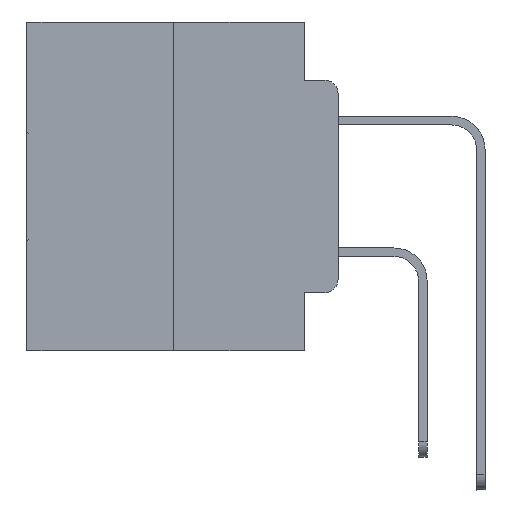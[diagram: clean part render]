
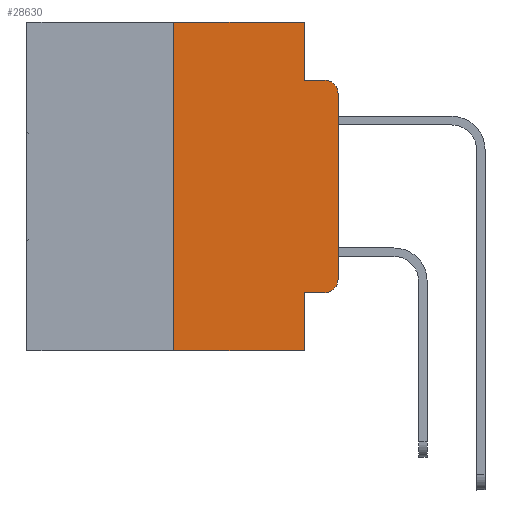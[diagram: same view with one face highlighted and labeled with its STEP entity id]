
A CAD part, left-side view. The second image highlights one B-rep face of the part: STEP entity #28630.
In plain terms, the highlighted planar face has unit normal (-1, 0, 0).
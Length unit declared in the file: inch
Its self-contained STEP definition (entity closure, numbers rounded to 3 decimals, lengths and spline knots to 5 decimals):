
#294 = DIRECTION ( 'NONE',  ( -1., 0., 0. ) ) ;
#558 = VECTOR ( 'NONE', #21208, 39.37008 ) ;
#645 = LINE ( 'NONE', #25226, #17899 ) ;
#706 = LINE ( 'NONE', #5748, #23135 ) ;
#824 = VERTEX_POINT ( 'NONE', #31595 ) ;
#925 = CARTESIAN_POINT ( 'NONE',  ( 0., 0.473, 0. ) ) ;
#1940 = VERTEX_POINT ( 'NONE', #3698 ) ;
#2618 = DIRECTION ( 'NONE',  ( 1., 0., 0. ) ) ;
#2751 = AXIS2_PLACEMENT_3D ( 'NONE', #14516, #294, #24709 ) ;
#2866 = AXIS2_PLACEMENT_3D ( 'NONE', #17154, #2618, #24914 ) ;
#2943 = ORIENTED_EDGE ( 'NONE', *, *, #8196, .T. ) ;
#3233 = CIRCLE ( 'NONE', #14081, 0.02 ) ;
#3653 = VECTOR ( 'NONE', #10638, 39.37008 ) ;
#3698 = CARTESIAN_POINT ( 'NONE',  ( 0., 0.25, 0. ) ) ;
#3915 = DIRECTION ( 'NONE',  ( -1., 0., 0. ) ) ;
#4068 = EDGE_CURVE ( 'NONE', #16028, #824, #706, .T. ) ;
#4870 = CARTESIAN_POINT ( 'NONE',  ( 0., 0.051, -0.0885 ) ) ;
#4882 = DIRECTION ( 'NONE',  ( 0., 0., 1. ) ) ;
#5057 = VERTEX_POINT ( 'NONE', #21976 ) ;
#5178 = VERTEX_POINT ( 'NONE', #8101 ) ;
#5705 = ORIENTED_EDGE ( 'NONE', *, *, #24037, .T. ) ;
#5748 = CARTESIAN_POINT ( 'NONE',  ( 0., 0.473, -0.5 ) ) ;
#5898 = DIRECTION ( 'NONE',  ( 0., 0., -1. ) ) ;
#5925 = CARTESIAN_POINT ( 'NONE',  ( 0., 0.02, -0.0885 ) ) ;
#6218 = LINE ( 'NONE', #25750, #27568 ) ;
#6695 = ORIENTED_EDGE ( 'NONE', *, *, #31089, .T. ) ;
#6992 = CARTESIAN_POINT ( 'NONE',  ( 0., 0.25, -0.5 ) ) ;
#8101 = CARTESIAN_POINT ( 'NONE',  ( 0., 0.02, -0.4115 ) ) ;
#8196 = EDGE_CURVE ( 'NONE', #5057, #30919, #21357, .T. ) ;
#8535 = DIRECTION ( 'NONE',  ( 0., -1., 0. ) ) ;
#8568 = LINE ( 'NONE', #925, #3653 ) ;
#8648 = CARTESIAN_POINT ( 'NONE',  ( 0., 0.051, 0. ) ) ;
#9656 = VECTOR ( 'NONE', #31451, 39.37008 ) ;
#10227 = LINE ( 'NONE', #20076, #31066 ) ;
#10367 = DIRECTION ( 'NONE',  ( 0., 0., 1. ) ) ;
#10483 = CARTESIAN_POINT ( 'NONE',  ( 0., 0.051, 0. ) ) ;
#10638 = DIRECTION ( 'NONE',  ( 0., -1., 0. ) ) ;
#10921 = LINE ( 'NONE', #20783, #17069 ) ;
#11357 = CARTESIAN_POINT ( 'NONE',  ( 0., 0.02, -0.3915 ) ) ;
#11668 = ORIENTED_EDGE ( 'NONE', *, *, #12736, .T. ) ;
#12736 = EDGE_CURVE ( 'NONE', #5178, #23157, #3233, .T. ) ;
#12981 = CARTESIAN_POINT ( 'NONE',  ( 0., 0., -0.3915 ) ) ;
#14081 = AXIS2_PLACEMENT_3D ( 'NONE', #11357, #3915, #21217 ) ;
#14516 = CARTESIAN_POINT ( 'NONE',  ( 0., 0.02, -0.1085 ) ) ;
#16028 = VERTEX_POINT ( 'NONE', #6992 ) ;
#16425 = LINE ( 'NONE', #31290, #9656 ) ;
#17069 = VECTOR ( 'NONE', #8535, 39.37008 ) ;
#17154 = CARTESIAN_POINT ( 'NONE',  ( 0., 0.473, 0. ) ) ;
#17899 = VECTOR ( 'NONE', #10367, 39.37008 ) ;
#18168 = EDGE_CURVE ( 'NONE', #19369, #30919, #16425, .T. ) ;
#19369 = VERTEX_POINT ( 'NONE', #4870 ) ;
#20076 = CARTESIAN_POINT ( 'NONE',  ( 0., 0.25, 0. ) ) ;
#20194 = ORIENTED_EDGE ( 'NONE', *, *, #24696, .F. ) ;
#20725 = LINE ( 'NONE', #8648, #558 ) ;
#20783 = CARTESIAN_POINT ( 'NONE',  ( 0., 0.051, -0.4115 ) ) ;
#20865 = ORIENTED_EDGE ( 'NONE', *, *, #18168, .F. ) ;
#21208 = DIRECTION ( 'NONE',  ( 0., 0., -1. ) ) ;
#21217 = DIRECTION ( 'NONE',  ( 0., 0., -1. ) ) ;
#21267 = EDGE_CURVE ( 'NONE', #31596, #19369, #20725, .T. ) ;
#21357 = CIRCLE ( 'NONE', #2751, 0.02 ) ;
#21976 = CARTESIAN_POINT ( 'NONE',  ( 0., 0., -0.1085 ) ) ;
#22282 = EDGE_CURVE ( 'NONE', #1940, #31596, #8568, .T. ) ;
#22968 = ORIENTED_EDGE ( 'NONE', *, *, #22282, .F. ) ;
#23135 = VECTOR ( 'NONE', #28324, 39.37008 ) ;
#23157 = VERTEX_POINT ( 'NONE', #12981 ) ;
#24037 = EDGE_CURVE ( 'NONE', #24691, #5178, #10921, .T. ) ;
#24691 = VERTEX_POINT ( 'NONE', #27494 ) ;
#24696 = EDGE_CURVE ( 'NONE', #16028, #1940, #10227, .T. ) ;
#24709 = DIRECTION ( 'NONE',  ( 0., 0., -1. ) ) ;
#24758 = PLANE ( 'NONE',  #2866 ) ;
#24914 = DIRECTION ( 'NONE',  ( 0., 0., -1. ) ) ;
#25226 = CARTESIAN_POINT ( 'NONE',  ( 0., 0., 0. ) ) ;
#25705 = ORIENTED_EDGE ( 'NONE', *, *, #21267, .F. ) ;
#25750 = CARTESIAN_POINT ( 'NONE',  ( 0., 0.051, 0. ) ) ;
#26987 = EDGE_CURVE ( 'NONE', #24691, #824, #6218, .T. ) ;
#27494 = CARTESIAN_POINT ( 'NONE',  ( 0., 0.051, -0.4115 ) ) ;
#27568 = VECTOR ( 'NONE', #5898, 39.37008 ) ;
#28324 = DIRECTION ( 'NONE',  ( 0., -1., 0. ) ) ;
#28630 = ADVANCED_FACE ( 'NONE', ( #30079 ), #24758, .F. ) ;
#29601 = ORIENTED_EDGE ( 'NONE', *, *, #4068, .T. ) ;
#29900 = EDGE_LOOP ( 'NONE', ( #6695, #2943, #20865, #25705, #22968, #20194, #29601, #30298, #5705, #11668 ) ) ;
#30079 = FACE_OUTER_BOUND ( 'NONE', #29900, .T. ) ;
#30298 = ORIENTED_EDGE ( 'NONE', *, *, #26987, .F. ) ;
#30919 = VERTEX_POINT ( 'NONE', #5925 ) ;
#31066 = VECTOR ( 'NONE', #4882, 39.37008 ) ;
#31089 = EDGE_CURVE ( 'NONE', #23157, #5057, #645, .T. ) ;
#31290 = CARTESIAN_POINT ( 'NONE',  ( 0., 0.051, -0.0885 ) ) ;
#31451 = DIRECTION ( 'NONE',  ( 0., -1., 0. ) ) ;
#31595 = CARTESIAN_POINT ( 'NONE',  ( 0., 0.051, -0.5 ) ) ;
#31596 = VERTEX_POINT ( 'NONE', #10483 ) ;
